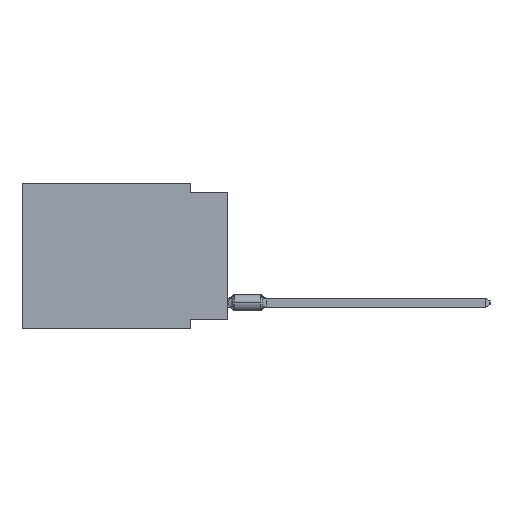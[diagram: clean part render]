
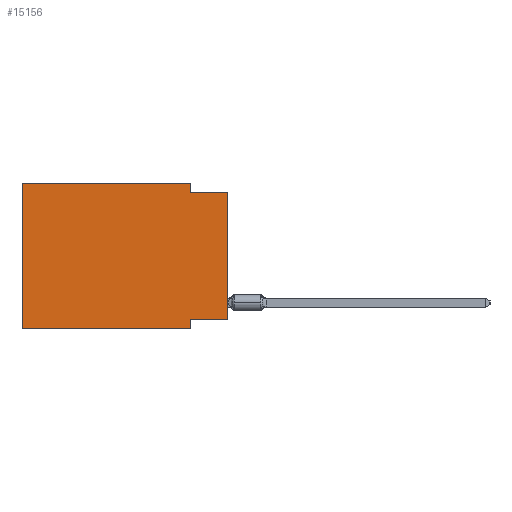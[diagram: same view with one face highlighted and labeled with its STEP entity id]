
A CAD part, left-side view. The second image highlights one B-rep face of the part: STEP entity #15156.
In plain terms, the highlighted planar face has unit normal (-1, 0, 0).
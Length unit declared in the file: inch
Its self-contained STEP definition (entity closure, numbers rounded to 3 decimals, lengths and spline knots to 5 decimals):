
#309 = EDGE_CURVE ( 'NONE', #60758, #23470, #15350, .T. ) ;
#702 = LINE ( 'NONE', #1592, #31788 ) ;
#1248 = ORIENTED_EDGE ( 'NONE', *, *, #17171, .F. ) ;
#1592 = CARTESIAN_POINT ( 'NONE',  ( 0., 0.1, 0. ) ) ;
#1818 = VECTOR ( 'NONE', #24558, 39.37008 ) ;
#2195 = VECTOR ( 'NONE', #40340, 39.37008 ) ;
#4097 = DIRECTION ( 'NONE',  ( 1., 0., 0. ) ) ;
#5901 = AXIS2_PLACEMENT_3D ( 'NONE', #12402, #4097, #50468 ) ;
#6251 = ORIENTED_EDGE ( 'NONE', *, *, #49352, .F. ) ;
#6720 = CARTESIAN_POINT ( 'NONE',  ( 0., 0., -0.025 ) ) ;
#8597 = EDGE_LOOP ( 'NONE', ( #13814, #47698, #48306, #35893, #44732, #39866, #1248, #6251 ) ) ;
#8771 = EDGE_CURVE ( 'NONE', #22778, #46945, #38713, .T. ) ;
#9841 = CARTESIAN_POINT ( 'NONE',  ( 0., 0., 0. ) ) ;
#10334 = CARTESIAN_POINT ( 'NONE',  ( 0., 0.55, 0. ) ) ;
#10968 = CARTESIAN_POINT ( 'NONE',  ( 0., 0., -0.025 ) ) ;
#12402 = CARTESIAN_POINT ( 'NONE',  ( 0., 0.55, 0. ) ) ;
#13814 = ORIENTED_EDGE ( 'NONE', *, *, #309, .T. ) ;
#14947 = CARTESIAN_POINT ( 'NONE',  ( 0., 0.1, -0.39 ) ) ;
#15156 = ADVANCED_FACE ( 'NONE', ( #17000 ), #44949, .F. ) ;
#15350 = LINE ( 'NONE', #9841, #1818 ) ;
#16002 = DIRECTION ( 'NONE',  ( 0., -1., 0. ) ) ;
#16167 = CARTESIAN_POINT ( 'NONE',  ( 0., 0.1, -0.025 ) ) ;
#17000 = FACE_OUTER_BOUND ( 'NONE', #8597, .T. ) ;
#17171 = EDGE_CURVE ( 'NONE', #59964, #46422, #40093, .T. ) ;
#18301 = CARTESIAN_POINT ( 'NONE',  ( 0., 0.1, -0.365 ) ) ;
#19572 = CARTESIAN_POINT ( 'NONE',  ( 0., 0.55, 0. ) ) ;
#22778 = VERTEX_POINT ( 'NONE', #10334 ) ;
#23470 = VERTEX_POINT ( 'NONE', #6720 ) ;
#24558 = DIRECTION ( 'NONE',  ( 0., 0., 1. ) ) ;
#25657 = CARTESIAN_POINT ( 'NONE',  ( 0., 0.1, -0.39 ) ) ;
#26129 = VECTOR ( 'NONE', #16002, 39.37008 ) ;
#28506 = VERTEX_POINT ( 'NONE', #58584 ) ;
#29649 = DIRECTION ( 'NONE',  ( 0., 0., -1. ) ) ;
#29680 = DIRECTION ( 'NONE',  ( 0., -1., 0. ) ) ;
#31711 = LINE ( 'NONE', #32323, #40327 ) ;
#31788 = VECTOR ( 'NONE', #52574, 39.37008 ) ;
#32323 = CARTESIAN_POINT ( 'NONE',  ( 0., 0.55, -0.39 ) ) ;
#32792 = DIRECTION ( 'NONE',  ( 0., 0., 1. ) ) ;
#34291 = LINE ( 'NONE', #10968, #52476 ) ;
#34631 = VECTOR ( 'NONE', #32792, 39.37008 ) ;
#35893 = ORIENTED_EDGE ( 'NONE', *, *, #8771, .F. ) ;
#37386 = LINE ( 'NONE', #19572, #34631 ) ;
#38713 = LINE ( 'NONE', #48863, #26129 ) ;
#39866 = ORIENTED_EDGE ( 'NONE', *, *, #46603, .T. ) ;
#40093 = LINE ( 'NONE', #25657, #54949 ) ;
#40327 = VECTOR ( 'NONE', #51065, 39.37008 ) ;
#40340 = DIRECTION ( 'NONE',  ( 0., 1., 0. ) ) ;
#40851 = CARTESIAN_POINT ( 'NONE',  ( 0., 0.1, 0. ) ) ;
#44732 = ORIENTED_EDGE ( 'NONE', *, *, #57742, .F. ) ;
#44949 = PLANE ( 'NONE',  #5901 ) ;
#46422 = VERTEX_POINT ( 'NONE', #14947 ) ;
#46603 = EDGE_CURVE ( 'NONE', #28506, #46422, #31711, .T. ) ;
#46945 = VERTEX_POINT ( 'NONE', #40851 ) ;
#47698 = ORIENTED_EDGE ( 'NONE', *, *, #59927, .F. ) ;
#48306 = ORIENTED_EDGE ( 'NONE', *, *, #57053, .F. ) ;
#48863 = CARTESIAN_POINT ( 'NONE',  ( 0., 0.55, 0. ) ) ;
#49352 = EDGE_CURVE ( 'NONE', #60758, #59964, #54177, .T. ) ;
#50468 = DIRECTION ( 'NONE',  ( 0., 0., -1. ) ) ;
#51065 = DIRECTION ( 'NONE',  ( 0., -1., 0. ) ) ;
#52476 = VECTOR ( 'NONE', #29680, 39.37008 ) ;
#52574 = DIRECTION ( 'NONE',  ( 0., 0., -1. ) ) ;
#53890 = VERTEX_POINT ( 'NONE', #16167 ) ;
#54177 = LINE ( 'NONE', #58799, #2195 ) ;
#54949 = VECTOR ( 'NONE', #29649, 39.37008 ) ;
#57053 = EDGE_CURVE ( 'NONE', #46945, #53890, #702, .T. ) ;
#57742 = EDGE_CURVE ( 'NONE', #28506, #22778, #37386, .T. ) ;
#58584 = CARTESIAN_POINT ( 'NONE',  ( 0., 0.55, -0.39 ) ) ;
#58660 = CARTESIAN_POINT ( 'NONE',  ( 0., 0., -0.365 ) ) ;
#58799 = CARTESIAN_POINT ( 'NONE',  ( 0., 0., -0.365 ) ) ;
#59927 = EDGE_CURVE ( 'NONE', #53890, #23470, #34291, .T. ) ;
#59964 = VERTEX_POINT ( 'NONE', #18301 ) ;
#60758 = VERTEX_POINT ( 'NONE', #58660 ) ;
